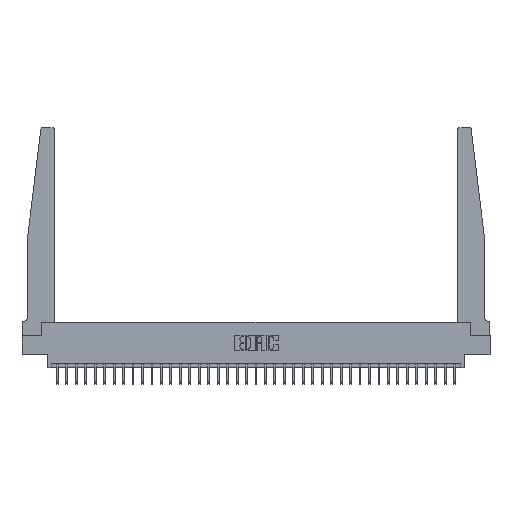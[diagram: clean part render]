
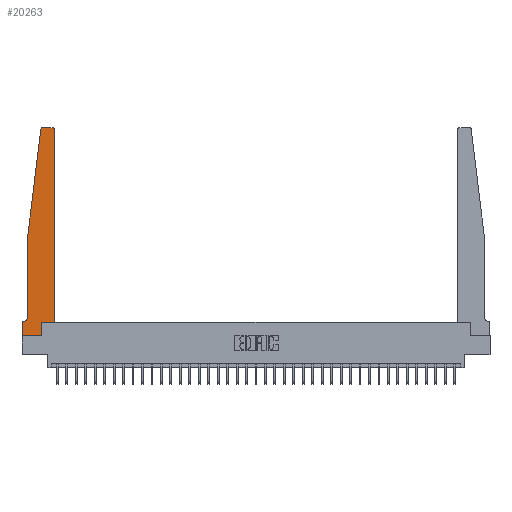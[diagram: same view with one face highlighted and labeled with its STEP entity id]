
A CAD part, top view. The second image highlights one B-rep face of the part: STEP entity #20263.
In plain terms, the highlighted planar face has unit normal (0, 0, 1).
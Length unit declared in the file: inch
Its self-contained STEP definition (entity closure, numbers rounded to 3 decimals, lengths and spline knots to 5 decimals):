
#95 = VERTEX_POINT ( 'NONE', #14993 ) ;
#317 = VERTEX_POINT ( 'NONE', #19814 ) ;
#649 = DIRECTION ( 'NONE',  ( -1., 0., 0. ) ) ;
#829 = EDGE_CURVE ( 'NONE', #22143, #31011, #31680, .T. ) ;
#1076 = CIRCLE ( 'NONE', #16426, 0.03 ) ;
#1656 = CARTESIAN_POINT ( 'NONE',  ( 0.425, 0.18, 0.37 ) ) ;
#2406 = ORIENTED_EDGE ( 'NONE', *, *, #3351, .T. ) ;
#2675 = AXIS2_PLACEMENT_3D ( 'NONE', #9813, #15739, #649 ) ;
#2702 = CARTESIAN_POINT ( 'NONE',  ( 0., 0.1875, 0.37 ) ) ;
#3351 = EDGE_CURVE ( 'NONE', #16452, #16007, #1076, .T. ) ;
#3811 = VECTOR ( 'NONE', #13140, 39.37008 ) ;
#3860 = DIRECTION ( 'NONE',  ( 1., 0., 0. ) ) ;
#3873 = EDGE_CURVE ( 'NONE', #19468, #24004, #28655, .T. ) ;
#4426 = EDGE_CURVE ( 'NONE', #19039, #317, #12272, .T. ) ;
#4657 = LINE ( 'NONE', #4833, #3811 ) ;
#4833 = CARTESIAN_POINT ( 'NONE',  ( 0.065, 0.1875, 0.37 ) ) ;
#4936 = EDGE_CURVE ( 'NONE', #24004, #16452, #7246, .T. ) ;
#6017 = DIRECTION ( 'NONE',  ( 0., 0., 1. ) ) ;
#6203 = ORIENTED_EDGE ( 'NONE', *, *, #15644, .T. ) ;
#6755 = ORIENTED_EDGE ( 'NONE', *, *, #4936, .T. ) ;
#7246 = LINE ( 'NONE', #24935, #22692 ) ;
#7506 = ORIENTED_EDGE ( 'NONE', *, *, #33159, .T. ) ;
#8648 = VECTOR ( 'NONE', #30640, 39.37008 ) ;
#8915 = CIRCLE ( 'NONE', #17679, 0.03 ) ;
#9648 = EDGE_CURVE ( 'NONE', #19674, #95, #25230, .T. ) ;
#9813 = CARTESIAN_POINT ( 'NONE',  ( 0.015, 0.2375, 0.37 ) ) ;
#9911 = EDGE_CURVE ( 'NONE', #30315, #22143, #8915, .T. ) ;
#10243 = CARTESIAN_POINT ( 'NONE',  ( 0.065, 1.25, 0.37 ) ) ;
#10337 = LINE ( 'NONE', #11840, #8648 ) ;
#10419 = CARTESIAN_POINT ( 'NONE',  ( 0.065, 0.2375, 0.37 ) ) ;
#10599 = CARTESIAN_POINT ( 'NONE',  ( 0.2605, 0.18, 0.37 ) ) ;
#11354 = ORIENTED_EDGE ( 'NONE', *, *, #3873, .T. ) ;
#11597 = CARTESIAN_POINT ( 'NONE',  ( 0.065, 1.25, 0.37 ) ) ;
#11710 = DIRECTION ( 'NONE',  ( -0.122, -0.992, 0. ) ) ;
#11840 = CARTESIAN_POINT ( 'NONE',  ( 0.065, 1.25, 0.37 ) ) ;
#12027 = AXIS2_PLACEMENT_3D ( 'NONE', #18048, #13027, #32407 ) ;
#12272 = LINE ( 'NONE', #30739, #31566 ) ;
#12674 = CARTESIAN_POINT ( 'NONE',  ( 0.425, 0.18, 0.37 ) ) ;
#12885 = ORIENTED_EDGE ( 'NONE', *, *, #829, .T. ) ;
#13027 = DIRECTION ( 'NONE',  ( 0., 0., 1. ) ) ;
#13097 = CARTESIAN_POINT ( 'NONE',  ( 0.24675, 2.72367, 0.37 ) ) ;
#13140 = DIRECTION ( 'NONE',  ( -1., 0., 0. ) ) ;
#13338 = DIRECTION ( 'NONE',  ( 0., 0., 1. ) ) ;
#13710 = LINE ( 'NONE', #16046, #19977 ) ;
#13745 = ORIENTED_EDGE ( 'NONE', *, *, #4426, .T. ) ;
#14799 = DIRECTION ( 'NONE',  ( 1., 0., 0. ) ) ;
#14993 = CARTESIAN_POINT ( 'NONE',  ( 0.015, 0.1875, 0.37 ) ) ;
#15621 = VECTOR ( 'NONE', #29286, 39.37008 ) ;
#15644 = EDGE_CURVE ( 'NONE', #317, #19468, #22234, .T. ) ;
#15739 = DIRECTION ( 'NONE',  ( 0., 0., -1. ) ) ;
#15995 = DIRECTION ( 'NONE',  ( 1., 0., 0. ) ) ;
#16007 = VERTEX_POINT ( 'NONE', #19042 ) ;
#16046 = CARTESIAN_POINT ( 'NONE',  ( 0.25, 2.75, 0.37 ) ) ;
#16426 = AXIS2_PLACEMENT_3D ( 'NONE', #29313, #13338, #15995 ) ;
#16452 = VERTEX_POINT ( 'NONE', #26318 ) ;
#16462 = ORIENTED_EDGE ( 'NONE', *, *, #25264, .T. ) ;
#16984 = DIRECTION ( 'NONE',  ( 0., 1., 0. ) ) ;
#17679 = AXIS2_PLACEMENT_3D ( 'NONE', #19110, #6017, #29991 ) ;
#18048 = CARTESIAN_POINT ( 'NONE',  ( 0., 0.1875, 0.37 ) ) ;
#18712 = ORIENTED_EDGE ( 'NONE', *, *, #28364, .T. ) ;
#19039 = VERTEX_POINT ( 'NONE', #25706 ) ;
#19042 = CARTESIAN_POINT ( 'NONE',  ( 0.395, 2.75, 0.37 ) ) ;
#19110 = CARTESIAN_POINT ( 'NONE',  ( 0.27653, 2.72, 0.37 ) ) ;
#19339 = VECTOR ( 'NONE', #16984, 39.37008 ) ;
#19468 = VERTEX_POINT ( 'NONE', #22645 ) ;
#19674 = VERTEX_POINT ( 'NONE', #10419 ) ;
#19814 = CARTESIAN_POINT ( 'NONE',  ( 0.2605, 0., 0.37 ) ) ;
#19924 = VECTOR ( 'NONE', #11710, 39.37008 ) ;
#19977 = VECTOR ( 'NONE', #24257, 39.37008 ) ;
#20263 = ADVANCED_FACE ( 'NONE', ( #23145 ), #21164, .T. ) ;
#20553 = EDGE_CURVE ( 'NONE', #27692, #19039, #26104, .T. ) ;
#20964 = ORIENTED_EDGE ( 'NONE', *, *, #20553, .T. ) ;
#21164 = PLANE ( 'NONE',  #12027 ) ;
#21496 = VECTOR ( 'NONE', #14799, 39.37008 ) ;
#22143 = VERTEX_POINT ( 'NONE', #13097 ) ;
#22234 = LINE ( 'NONE', #10599, #19339 ) ;
#22645 = CARTESIAN_POINT ( 'NONE',  ( 0.2605, 0.18, 0.37 ) ) ;
#22692 = VECTOR ( 'NONE', #33675, 39.37008 ) ;
#23145 = FACE_OUTER_BOUND ( 'NONE', #24560, .T. ) ;
#24004 = VERTEX_POINT ( 'NONE', #1656 ) ;
#24257 = DIRECTION ( 'NONE',  ( -1., 0., 0. ) ) ;
#24560 = EDGE_LOOP ( 'NONE', ( #7506, #29683, #12885, #18712, #27099, #16462, #20964, #13745, #6203, #11354, #6755, #2406 ) ) ;
#24935 = CARTESIAN_POINT ( 'NONE',  ( 0.425, 0.18, 0.37 ) ) ;
#25230 = CIRCLE ( 'NONE', #2675, 0.05 ) ;
#25264 = EDGE_CURVE ( 'NONE', #95, #27692, #4657, .T. ) ;
#25706 = CARTESIAN_POINT ( 'NONE',  ( 0., 0., 0.37 ) ) ;
#26065 = CARTESIAN_POINT ( 'NONE',  ( 0.27653, 2.75, 0.37 ) ) ;
#26104 = LINE ( 'NONE', #31910, #15621 ) ;
#26318 = CARTESIAN_POINT ( 'NONE',  ( 0.425, 2.72, 0.37 ) ) ;
#27099 = ORIENTED_EDGE ( 'NONE', *, *, #9648, .T. ) ;
#27692 = VERTEX_POINT ( 'NONE', #2702 ) ;
#28364 = EDGE_CURVE ( 'NONE', #31011, #19674, #10337, .T. ) ;
#28655 = LINE ( 'NONE', #12674, #21496 ) ;
#29286 = DIRECTION ( 'NONE',  ( 0., -1., 0. ) ) ;
#29313 = CARTESIAN_POINT ( 'NONE',  ( 0.395, 2.72, 0.37 ) ) ;
#29683 = ORIENTED_EDGE ( 'NONE', *, *, #9911, .T. ) ;
#29991 = DIRECTION ( 'NONE',  ( 1., 0., 0. ) ) ;
#30315 = VERTEX_POINT ( 'NONE', #26065 ) ;
#30640 = DIRECTION ( 'NONE',  ( 0., -1., 0. ) ) ;
#30739 = CARTESIAN_POINT ( 'NONE',  ( 0., 0., 0.37 ) ) ;
#31011 = VERTEX_POINT ( 'NONE', #10243 ) ;
#31566 = VECTOR ( 'NONE', #3860, 39.37008 ) ;
#31680 = LINE ( 'NONE', #11597, #19924 ) ;
#31910 = CARTESIAN_POINT ( 'NONE',  ( 0., 0., 0.37 ) ) ;
#32407 = DIRECTION ( 'NONE',  ( 1., 0., 0. ) ) ;
#33159 = EDGE_CURVE ( 'NONE', #16007, #30315, #13710, .T. ) ;
#33675 = DIRECTION ( 'NONE',  ( 0., 1., 0. ) ) ;
